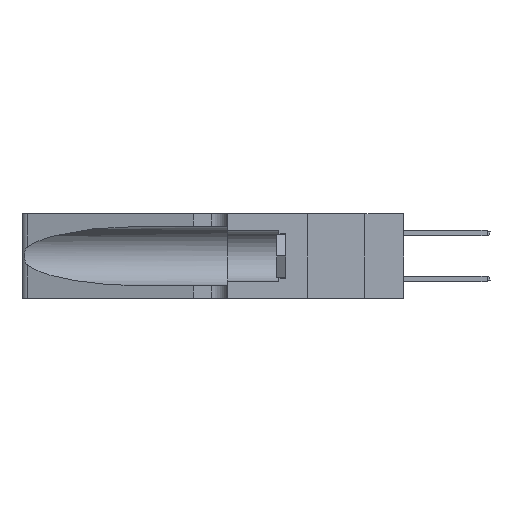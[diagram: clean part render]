
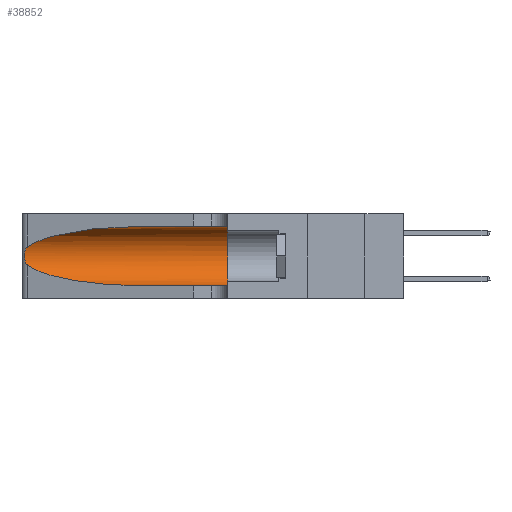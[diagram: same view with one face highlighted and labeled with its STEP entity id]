
A CAD part, left-side view. The second image highlights one B-rep face of the part: STEP entity #38852.
In plain terms, the highlighted cylindrical face has radius 3.308 mm (diameter 6.617 mm), a partial arc.
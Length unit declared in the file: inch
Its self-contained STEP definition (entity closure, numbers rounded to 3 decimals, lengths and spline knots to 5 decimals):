
#480 = ORIENTED_EDGE ( 'NONE', *, *, #16018, .T. ) ;
#959 = CARTESIAN_POINT ( 'NONE',  ( 0.25787, 1.23484, 0.2124 ) ) ;
#2684 = EDGE_CURVE ( 'NONE', #4892, #21665, #40591, .T. ) ;
#3364 = DIRECTION ( 'NONE',  ( 0., 1., 0. ) ) ;
#4405 = CARTESIAN_POINT ( 'NONE',  ( 0.26075, 1.23896, 0.178 ) ) ;
#4892 = VERTEX_POINT ( 'NONE', #28201 ) ;
#4956 = CARTESIAN_POINT ( 'NONE',  ( 0.1305, 0.72297, 0.05475 ) ) ;
#5033 = CARTESIAN_POINT ( 'NONE',  ( 0.25555, 1.22994, 0.2215 ) ) ;
#5523 = CARTESIAN_POINT ( 'NONE',  ( 0.2373, 1.15595, 0.28018 ) ) ;
#5721 =( BOUNDED_CURVE ( )  B_SPLINE_CURVE ( 3, ( #6120, #20230, #5523, #34136 ),
 .UNSPECIFIED., .F., .F. ) 
 B_SPLINE_CURVE_WITH_KNOTS ( ( 4, 4 ),
 ( 1.5708, 2.84003 ),
 .UNSPECIFIED. ) 
 CURVE ( )  GEOMETRIC_REPRESENTATION_ITEM ( )  RATIONAL_B_SPLINE_CURVE ( ( 1., 0.87, 0.87, 1. ) ) 
 REPRESENTATION_ITEM ( '' )  );
#6120 = CARTESIAN_POINT ( 'NONE',  ( 0.1305, 0.72297, 0.31525 ) ) ;
#6549 = FACE_OUTER_BOUND ( 'NONE', #18693, .T. ) ;
#8244 = CARTESIAN_POINT ( 'NONE',  ( 0.18966, 0.96281, 0.05475 ) ) ;
#9224 = CARTESIAN_POINT ( 'NONE',  ( 0.25789, 1.23486, 0.15765 ) ) ;
#11091 = VECTOR ( 'NONE', #30471, 39.37008 ) ;
#11276 = ORIENTED_EDGE ( 'NONE', *, *, #45512, .T. ) ;
#11722 = CARTESIAN_POINT ( 'NONE',  ( 0.1305, 0.72297, 0.05475 ) ) ;
#11968 = ORIENTED_EDGE ( 'NONE', *, *, #13336, .F. ) ;
#13336 = EDGE_CURVE ( 'NONE', #21665, #26176, #19651, .T. ) ;
#14525 = CARTESIAN_POINT ( 'NONE',  ( 0.1305, 0.35, 0.185 ) ) ;
#14830 = VERTEX_POINT ( 'NONE', #11722 ) ;
#15705 = AXIS2_PLACEMENT_3D ( 'NONE', #28803, #32685, #39829 ) ;
#16018 = EDGE_CURVE ( 'NONE', #22116, #14830, #25815, .T. ) ;
#16072 = CARTESIAN_POINT ( 'NONE',  ( 0.1305, 1.61858, 0.05475 ) ) ;
#16590 = CARTESIAN_POINT ( 'NONE',  ( 0.1305, 0.35, 0.31525 ) ) ;
#16946 = EDGE_CURVE ( 'NONE', #4892, #21433, #5721, .T. ) ;
#18656 = CARTESIAN_POINT ( 'NONE',  ( 0.25639, 1.23184, 0.21858 ) ) ;
#18693 = EDGE_LOOP ( 'NONE', ( #39138, #40457, #480, #11276, #11968, #33451 ) ) ;
#19444 = CARTESIAN_POINT ( 'NONE',  ( 0.25555, 1.22993, 0.14849 ) ) ;
#19651 = CIRCLE ( 'NONE', #27671, 0.13025 ) ;
#20230 = CARTESIAN_POINT ( 'NONE',  ( 0.18966, 0.96281, 0.31525 ) ) ;
#21433 = VERTEX_POINT ( 'NONE', #37040 ) ;
#21665 = VERTEX_POINT ( 'NONE', #16590 ) ;
#22116 = VERTEX_POINT ( 'NONE', #30156 ) ;
#22354 = CARTESIAN_POINT ( 'NONE',  ( 0.2373, 1.15595, 0.08982 ) ) ;
#22584 = CARTESIAN_POINT ( 'NONE',  ( 0.25854, 1.2359, 0.20912 ) ) ;
#23648 = CARTESIAN_POINT ( 'NONE',  ( 0.25639, 1.23186, 0.15144 ) ) ;
#25815 =( BOUNDED_CURVE ( )  B_SPLINE_CURVE ( 3, ( #29731, #22354, #8244, #4956 ),
 .UNSPECIFIED., .F., .F. ) 
 B_SPLINE_CURVE_WITH_KNOTS ( ( 4, 4 ),
 ( 3.44316, 4.71239 ),
 .UNSPECIFIED. ) 
 CURVE ( )  GEOMETRIC_REPRESENTATION_ITEM ( )  RATIONAL_B_SPLINE_CURVE ( ( 1., 0.87, 0.87, 1. ) ) 
 REPRESENTATION_ITEM ( '' )  );
#25852 = CARTESIAN_POINT ( 'NONE',  ( 0.26075, 1.23896, 0.19203 ) ) ;
#26176 = VERTEX_POINT ( 'NONE', #45331 ) ;
#26481 = CARTESIAN_POINT ( 'NONE',  ( 0.25487, 1.22718, 0.22369 ) ) ;
#26948 = CARTESIAN_POINT ( 'NONE',  ( 0.26017, 1.23833, 0.17102 ) ) ;
#27671 = AXIS2_PLACEMENT_3D ( 'NONE', #14525, #3364, #28459 ) ;
#28201 = CARTESIAN_POINT ( 'NONE',  ( 0.1305, 0.72297, 0.31525 ) ) ;
#28459 = DIRECTION ( 'NONE',  ( 0., 0., 1. ) ) ;
#28803 = CARTESIAN_POINT ( 'NONE',  ( 0.1305, 1.61858, 0.185 ) ) ;
#29010 = CYLINDRICAL_SURFACE ( 'NONE', #15705, 0.13025 ) ;
#29731 = CARTESIAN_POINT ( 'NONE',  ( 0.25487, 1.22718, 0.14631 ) ) ;
#30156 = CARTESIAN_POINT ( 'NONE',  ( 0.25487, 1.22718, 0.14631 ) ) ;
#30471 = DIRECTION ( 'NONE',  ( 0., -1., 0. ) ) ;
#32685 = DIRECTION ( 'NONE',  ( 0., -1., 0. ) ) ;
#33451 = ORIENTED_EDGE ( 'NONE', *, *, #2684, .F. ) ;
#33497 = LINE ( 'NONE', #16072, #11091 ) ;
#33958 = CARTESIAN_POINT ( 'NONE',  ( 0.25487, 1.22718, 0.14631 ) ) ;
#34136 = CARTESIAN_POINT ( 'NONE',  ( 0.25487, 1.22718, 0.22369 ) ) ;
#36329 = CARTESIAN_POINT ( 'NONE',  ( 0.1305, 1.61858, 0.31525 ) ) ;
#37040 = CARTESIAN_POINT ( 'NONE',  ( 0.25487, 1.22718, 0.22369 ) ) ;
#38852 = ADVANCED_FACE ( 'NONE', ( #6549 ), #29010, .F. ) ;
#38857 = VECTOR ( 'NONE', #43541, 39.37008 ) ;
#39138 = ORIENTED_EDGE ( 'NONE', *, *, #16946, .T. ) ;
#39829 = DIRECTION ( 'NONE',  ( 0., 0., -1. ) ) ;
#40457 = ORIENTED_EDGE ( 'NONE', *, *, #44287, .T. ) ;
#40591 = LINE ( 'NONE', #36329, #38857 ) ;
#40975 = CARTESIAN_POINT ( 'NONE',  ( 0.25856, 1.23593, 0.16098 ) ) ;
#43541 = DIRECTION ( 'NONE',  ( 0., -1., 0. ) ) ;
#43665 = CARTESIAN_POINT ( 'NONE',  ( 0.26018, 1.23835, 0.19895 ) ) ;
#44287 = EDGE_CURVE ( 'NONE', #21433, #22116, #46134, .T. ) ;
#45331 = CARTESIAN_POINT ( 'NONE',  ( 0.1305, 0.35, 0.05475 ) ) ;
#45512 = EDGE_CURVE ( 'NONE', #14830, #26176, #33497, .T. ) ;
#46134 = B_SPLINE_CURVE_WITH_KNOTS ( 'NONE', 3,
 ( #26481, #5033, #18656, #959, #22584, #43665, #25852, #4405, #26948, #40975, #9224, #23648, #19444, #33958 ),
 .UNSPECIFIED., .F., .F.,
 ( 4, 2, 2, 2, 2, 2, 4 ),
 ( 0., 0.00027, 0.00053, 0.00107, 0.0016, 0.00187, 0.00214 ),
 .UNSPECIFIED. ) ;
